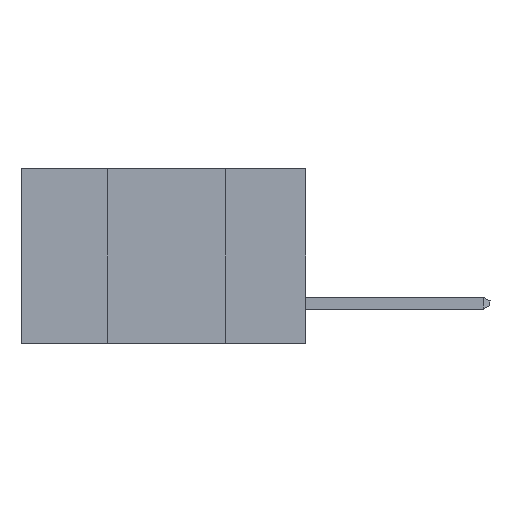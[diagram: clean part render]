
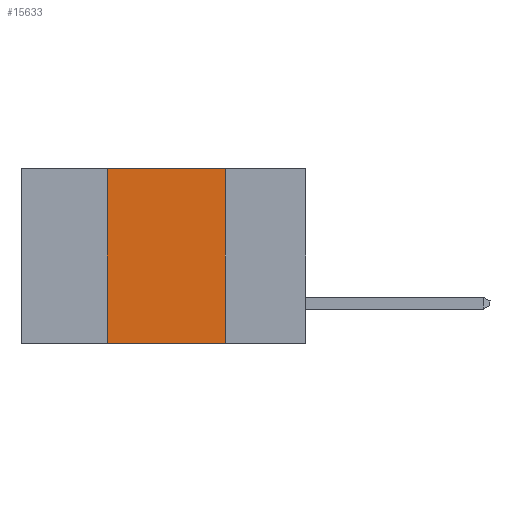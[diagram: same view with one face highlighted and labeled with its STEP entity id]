
A CAD part, left-side view. The second image highlights one B-rep face of the part: STEP entity #15633.
In plain terms, the highlighted planar face has unit normal (-1, 0, 0).
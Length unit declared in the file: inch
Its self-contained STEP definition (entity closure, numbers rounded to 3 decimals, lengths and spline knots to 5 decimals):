
#154 = DIRECTION ( 'NONE',  ( 0., -1., 0. ) ) ;
#348 = VERTEX_POINT ( 'NONE', #18284 ) ;
#1600 = CARTESIAN_POINT ( 'NONE',  ( 0., 0.6, -0.37 ) ) ;
#1701 = DIRECTION ( 'NONE',  ( 1., 0., 0. ) ) ;
#3168 = ORIENTED_EDGE ( 'NONE', *, *, #10415, .F. ) ;
#3477 = FACE_OUTER_BOUND ( 'NONE', #10738, .T. ) ;
#3615 = CARTESIAN_POINT ( 'NONE',  ( 0., 0.17, -0.37 ) ) ;
#4820 = VECTOR ( 'NONE', #6009, 39.37008 ) ;
#4969 = ORIENTED_EDGE ( 'NONE', *, *, #15101, .F. ) ;
#5628 = ORIENTED_EDGE ( 'NONE', *, *, #15783, .T. ) ;
#6009 = DIRECTION ( 'NONE',  ( 0., 0., 1. ) ) ;
#7680 = CARTESIAN_POINT ( 'NONE',  ( 0., 0.17, 0. ) ) ;
#8082 = ORIENTED_EDGE ( 'NONE', *, *, #21175, .F. ) ;
#8891 = PLANE ( 'NONE',  #9719 ) ;
#9719 = AXIS2_PLACEMENT_3D ( 'NONE', #14047, #1701, #12170 ) ;
#10219 = CARTESIAN_POINT ( 'NONE',  ( 0., 0.42, 0. ) ) ;
#10415 = EDGE_CURVE ( 'NONE', #348, #21480, #16657, .T. ) ;
#10738 = EDGE_LOOP ( 'NONE', ( #8082, #4969, #3168, #5628 ) ) ;
#11581 = VECTOR ( 'NONE', #14902, 39.37008 ) ;
#11936 = VECTOR ( 'NONE', #154, 39.37008 ) ;
#12170 = DIRECTION ( 'NONE',  ( 0., 0., -1. ) ) ;
#14047 = CARTESIAN_POINT ( 'NONE',  ( 0., 0.6, 0. ) ) ;
#14731 = CARTESIAN_POINT ( 'NONE',  ( 0., 0.42, 0. ) ) ;
#14902 = DIRECTION ( 'NONE',  ( 0., 0., -1. ) ) ;
#15101 = EDGE_CURVE ( 'NONE', #21480, #20030, #22117, .T. ) ;
#15633 = ADVANCED_FACE ( 'NONE', ( #3477 ), #8891, .F. ) ;
#15783 = EDGE_CURVE ( 'NONE', #348, #17608, #21217, .T. ) ;
#16213 = CARTESIAN_POINT ( 'NONE',  ( 0., 0.6, 0. ) ) ;
#16389 = LINE ( 'NONE', #7680, #11581 ) ;
#16424 = VECTOR ( 'NONE', #21373, 39.37008 ) ;
#16657 = LINE ( 'NONE', #14731, #4820 ) ;
#17608 = VERTEX_POINT ( 'NONE', #3615 ) ;
#18284 = CARTESIAN_POINT ( 'NONE',  ( 0., 0.42, -0.37 ) ) ;
#20030 = VERTEX_POINT ( 'NONE', #23066 ) ;
#21175 = EDGE_CURVE ( 'NONE', #20030, #17608, #16389, .T. ) ;
#21217 = LINE ( 'NONE', #1600, #16424 ) ;
#21373 = DIRECTION ( 'NONE',  ( 0., -1., 0. ) ) ;
#21480 = VERTEX_POINT ( 'NONE', #10219 ) ;
#22117 = LINE ( 'NONE', #16213, #11936 ) ;
#23066 = CARTESIAN_POINT ( 'NONE',  ( 0., 0.17, 0. ) ) ;
